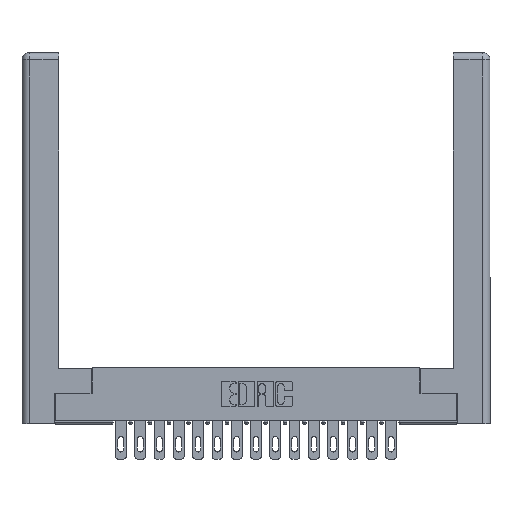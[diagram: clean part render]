
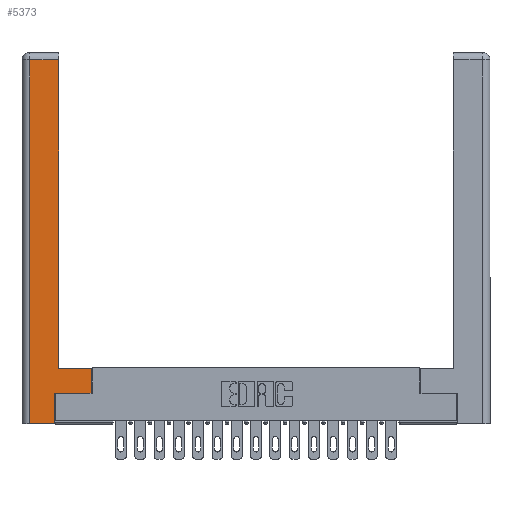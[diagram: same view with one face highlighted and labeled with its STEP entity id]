
A CAD part, top view. The second image highlights one B-rep face of the part: STEP entity #5373.
In plain terms, the highlighted planar face has unit normal (0, 0, 1).
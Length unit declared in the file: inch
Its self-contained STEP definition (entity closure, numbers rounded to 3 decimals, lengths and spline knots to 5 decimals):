
#291 = CARTESIAN_POINT ( 'NONE',  ( 0.295, 2.94, 0. ) ) ;
#550 = CARTESIAN_POINT ( 'NONE',  ( 0.0615, 0., 0. ) ) ;
#734 = EDGE_CURVE ( 'NONE', #15867, #12586, #16820, .T. ) ;
#803 = DIRECTION ( 'NONE',  ( -1., 0., 0. ) ) ;
#1561 = DIRECTION ( 'NONE',  ( 0., 1., 0. ) ) ;
#1643 = CARTESIAN_POINT ( 'NONE',  ( 0.565, 0.45, 0. ) ) ;
#1708 = CARTESIAN_POINT ( 'NONE',  ( 0.565, 0.45, 0. ) ) ;
#2247 = LINE ( 'NONE', #1643, #9590 ) ;
#2722 = CARTESIAN_POINT ( 'NONE',  ( 0.265, 0.245, 0. ) ) ;
#3227 = ORIENTED_EDGE ( 'NONE', *, *, #14998, .T. ) ;
#3330 = PLANE ( 'NONE',  #16775 ) ;
#3387 = EDGE_CURVE ( 'NONE', #12017, #11726, #2247, .T. ) ;
#3458 = ORIENTED_EDGE ( 'NONE', *, *, #3387, .T. ) ;
#4929 = DIRECTION ( 'NONE',  ( 0., 0., -1. ) ) ;
#5272 = CARTESIAN_POINT ( 'NONE',  ( 0.0615, 2.94, 0. ) ) ;
#5373 = ADVANCED_FACE ( 'NONE', ( #11952 ), #3330, .F. ) ;
#6027 = VECTOR ( 'NONE', #1561, 39.37008 ) ;
#6281 = VECTOR ( 'NONE', #20218, 39.37008 ) ;
#6741 = EDGE_CURVE ( 'NONE', #11726, #10482, #19205, .T. ) ;
#6806 = DIRECTION ( 'NONE',  ( 0., -1., 0. ) ) ;
#6914 = LINE ( 'NONE', #10904, #17892 ) ;
#7017 = EDGE_CURVE ( 'NONE', #10482, #9020, #11123, .T. ) ;
#7040 = EDGE_LOOP ( 'NONE', ( #11526, #13475, #17082, #13221, #3227, #19072, #3458, #16008 ) ) ;
#7067 = DIRECTION ( 'NONE',  ( 1., 0., 0. ) ) ;
#7574 = CARTESIAN_POINT ( 'NONE',  ( 0.265, 0., 0. ) ) ;
#8535 = CARTESIAN_POINT ( 'NONE',  ( 0.565, 0.245, 0. ) ) ;
#8669 = EDGE_CURVE ( 'NONE', #12586, #11031, #13326, .T. ) ;
#9020 = VERTEX_POINT ( 'NONE', #291 ) ;
#9329 = LINE ( 'NONE', #11671, #13040 ) ;
#9471 = EDGE_CURVE ( 'NONE', #13691, #12017, #6914, .T. ) ;
#9590 = VECTOR ( 'NONE', #18467, 39.37008 ) ;
#9774 = EDGE_CURVE ( 'NONE', #9020, #15867, #9329, .T. ) ;
#10078 = DIRECTION ( 'NONE',  ( -1., 0., 0. ) ) ;
#10196 = CARTESIAN_POINT ( 'NONE',  ( 0.295, 0.45, 0. ) ) ;
#10482 = VERTEX_POINT ( 'NONE', #16509 ) ;
#10873 = CARTESIAN_POINT ( 'NONE',  ( 0.265, 0.245, 0. ) ) ;
#10898 = LINE ( 'NONE', #10873, #6281 ) ;
#10904 = CARTESIAN_POINT ( 'NONE',  ( 0.565, 0.245, 0. ) ) ;
#11031 = VERTEX_POINT ( 'NONE', #7574 ) ;
#11123 = LINE ( 'NONE', #20284, #6027 ) ;
#11526 = ORIENTED_EDGE ( 'NONE', *, *, #7017, .T. ) ;
#11671 = CARTESIAN_POINT ( 'NONE',  ( 0.0615, 2.94, 0. ) ) ;
#11726 = VERTEX_POINT ( 'NONE', #1708 ) ;
#11915 = CARTESIAN_POINT ( 'NONE',  ( 0.0615, 0., 0. ) ) ;
#11952 = FACE_OUTER_BOUND ( 'NONE', #7040, .T. ) ;
#12017 = VERTEX_POINT ( 'NONE', #8535 ) ;
#12586 = VERTEX_POINT ( 'NONE', #550 ) ;
#12684 = VECTOR ( 'NONE', #6806, 39.37008 ) ;
#13040 = VECTOR ( 'NONE', #10078, 39.37008 ) ;
#13221 = ORIENTED_EDGE ( 'NONE', *, *, #8669, .T. ) ;
#13326 = LINE ( 'NONE', #16434, #16981 ) ;
#13475 = ORIENTED_EDGE ( 'NONE', *, *, #9774, .T. ) ;
#13691 = VERTEX_POINT ( 'NONE', #2722 ) ;
#14314 = CARTESIAN_POINT ( 'NONE',  ( 0., 0., 0. ) ) ;
#14593 = VECTOR ( 'NONE', #803, 39.37008 ) ;
#14998 = EDGE_CURVE ( 'NONE', #11031, #13691, #10898, .T. ) ;
#15867 = VERTEX_POINT ( 'NONE', #5272 ) ;
#15887 = DIRECTION ( 'NONE',  ( -1., 0., 0. ) ) ;
#16008 = ORIENTED_EDGE ( 'NONE', *, *, #6741, .T. ) ;
#16434 = CARTESIAN_POINT ( 'NONE',  ( 0.265, 0., 0. ) ) ;
#16509 = CARTESIAN_POINT ( 'NONE',  ( 0.295, 0.45, 0. ) ) ;
#16775 = AXIS2_PLACEMENT_3D ( 'NONE', #14314, #4929, #15887 ) ;
#16820 = LINE ( 'NONE', #11915, #12684 ) ;
#16981 = VECTOR ( 'NONE', #7067, 39.37008 ) ;
#17082 = ORIENTED_EDGE ( 'NONE', *, *, #734, .T. ) ;
#17892 = VECTOR ( 'NONE', #18716, 39.37008 ) ;
#18467 = DIRECTION ( 'NONE',  ( 0., 1., 0. ) ) ;
#18716 = DIRECTION ( 'NONE',  ( 1., 0., 0. ) ) ;
#19072 = ORIENTED_EDGE ( 'NONE', *, *, #9471, .T. ) ;
#19205 = LINE ( 'NONE', #10196, #14593 ) ;
#20218 = DIRECTION ( 'NONE',  ( 0., 1., 0. ) ) ;
#20284 = CARTESIAN_POINT ( 'NONE',  ( 0.295, 3., 0. ) ) ;
